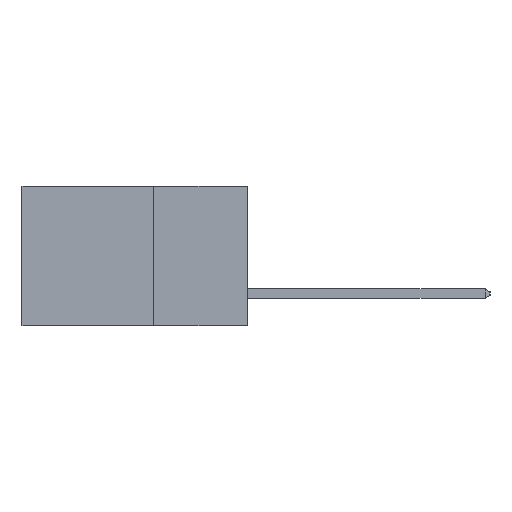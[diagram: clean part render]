
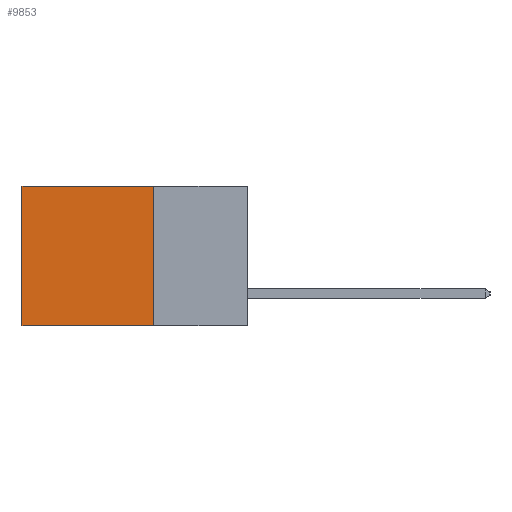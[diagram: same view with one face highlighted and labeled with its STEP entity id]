
A CAD part, left-side view. The second image highlights one B-rep face of the part: STEP entity #9853.
In plain terms, the highlighted planar face has unit normal (-1, 0, 0).
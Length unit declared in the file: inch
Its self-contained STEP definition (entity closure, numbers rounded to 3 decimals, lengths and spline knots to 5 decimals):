
#106 = EDGE_CURVE ( 'NONE', #6107, #361, #4923, .T. ) ;
#190 = VECTOR ( 'NONE', #1836, 39.37008 ) ;
#361 = VERTEX_POINT ( 'NONE', #682 ) ;
#682 = CARTESIAN_POINT ( 'NONE',  ( 0.298, 0.25, -0.37 ) ) ;
#886 = ORIENTED_EDGE ( 'NONE', *, *, #7646, .F. ) ;
#1700 = EDGE_CURVE ( 'NONE', #6107, #6439, #3127, .T. ) ;
#1836 = DIRECTION ( 'NONE',  ( 0., 1., 0. ) ) ;
#1870 = CARTESIAN_POINT ( 'NONE',  ( 0.298, 0.25, 0. ) ) ;
#1934 = DIRECTION ( 'NONE',  ( 0., 0., -1. ) ) ;
#1972 = DIRECTION ( 'NONE',  ( 0., 0., -1. ) ) ;
#2097 = CARTESIAN_POINT ( 'NONE',  ( 0.298, 0.25, 0. ) ) ;
#2161 = EDGE_LOOP ( 'NONE', ( #4066, #886, #6373, #7967 ) ) ;
#2430 = LINE ( 'NONE', #8983, #190 ) ;
#2803 = VECTOR ( 'NONE', #1972, 39.37008 ) ;
#3127 = LINE ( 'NONE', #2097, #9199 ) ;
#3458 = CARTESIAN_POINT ( 'NONE',  ( 0.298, 0.6, 0. ) ) ;
#4066 = ORIENTED_EDGE ( 'NONE', *, *, #7689, .T. ) ;
#4460 = CARTESIAN_POINT ( 'NONE',  ( 0.298, 0.6, -0.37 ) ) ;
#4923 = LINE ( 'NONE', #1870, #2803 ) ;
#5117 = PLANE ( 'NONE',  #9386 ) ;
#5937 = CARTESIAN_POINT ( 'NONE',  ( 0.298, 0.25, 0. ) ) ;
#5940 = DIRECTION ( 'NONE',  ( 0., 0., -1. ) ) ;
#5943 = VECTOR ( 'NONE', #5940, 39.37008 ) ;
#6107 = VERTEX_POINT ( 'NONE', #8657 ) ;
#6340 = FACE_OUTER_BOUND ( 'NONE', #2161, .T. ) ;
#6373 = ORIENTED_EDGE ( 'NONE', *, *, #106, .F. ) ;
#6439 = VERTEX_POINT ( 'NONE', #3458 ) ;
#6739 = DIRECTION ( 'NONE',  ( 1., 0., 0. ) ) ;
#7516 = CARTESIAN_POINT ( 'NONE',  ( 0.298, 0.6, 0. ) ) ;
#7646 = EDGE_CURVE ( 'NONE', #361, #8272, #2430, .T. ) ;
#7689 = EDGE_CURVE ( 'NONE', #6439, #8272, #8035, .T. ) ;
#7967 = ORIENTED_EDGE ( 'NONE', *, *, #1700, .T. ) ;
#8035 = LINE ( 'NONE', #7516, #5943 ) ;
#8272 = VERTEX_POINT ( 'NONE', #4460 ) ;
#8289 = DIRECTION ( 'NONE',  ( 0., 1., 0. ) ) ;
#8657 = CARTESIAN_POINT ( 'NONE',  ( 0.298, 0.25, 0. ) ) ;
#8983 = CARTESIAN_POINT ( 'NONE',  ( 0.298, 0.25, -0.37 ) ) ;
#9199 = VECTOR ( 'NONE', #8289, 39.37008 ) ;
#9386 = AXIS2_PLACEMENT_3D ( 'NONE', #5937, #6739, #1934 ) ;
#9853 = ADVANCED_FACE ( 'NONE', ( #6340 ), #5117, .F. ) ;
